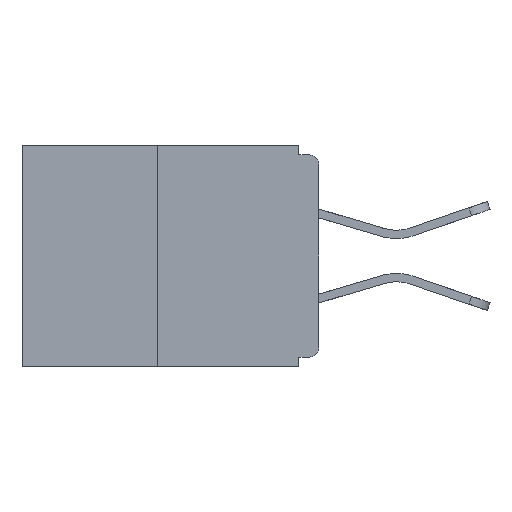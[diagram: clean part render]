
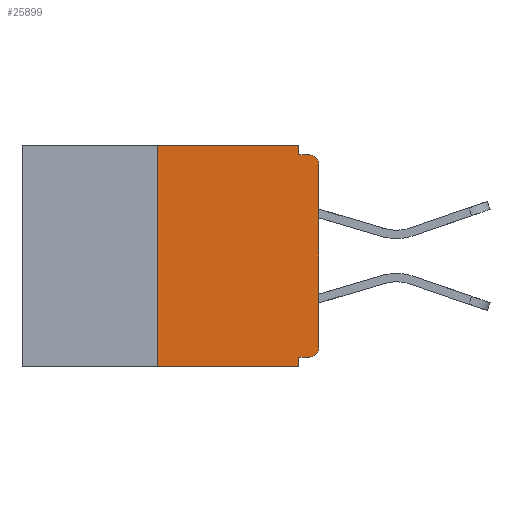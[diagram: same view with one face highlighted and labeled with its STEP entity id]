
A CAD part, left-side view. The second image highlights one B-rep face of the part: STEP entity #25899.
In plain terms, the highlighted planar face has unit normal (-1, 0, 0).
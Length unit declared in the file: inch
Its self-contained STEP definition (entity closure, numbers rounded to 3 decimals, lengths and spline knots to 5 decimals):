
#521 = EDGE_CURVE ( 'NONE', #12329, #2806, #24300, .T. ) ;
#1174 = VECTOR ( 'NONE', #25346, 39.37008 ) ;
#1480 = FACE_OUTER_BOUND ( 'NONE', #10178, .T. ) ;
#1652 = LINE ( 'NONE', #28042, #18317 ) ;
#1727 = DIRECTION ( 'NONE',  ( 0., 0., -1. ) ) ;
#1954 = DIRECTION ( 'NONE',  ( 0., -1., 0. ) ) ;
#2052 = CARTESIAN_POINT ( 'NONE',  ( 0., 0.25, 0. ) ) ;
#2169 = CARTESIAN_POINT ( 'NONE',  ( 0., 0.015, -0.313 ) ) ;
#2304 = ORIENTED_EDGE ( 'NONE', *, *, #11533, .F. ) ;
#2383 = ORIENTED_EDGE ( 'NONE', *, *, #22090, .F. ) ;
#2662 = VECTOR ( 'NONE', #10454, 39.37008 ) ;
#2806 = VERTEX_POINT ( 'NONE', #19488 ) ;
#2908 = LINE ( 'NONE', #6083, #15517 ) ;
#3956 = VERTEX_POINT ( 'NONE', #2052 ) ;
#6083 = CARTESIAN_POINT ( 'NONE',  ( 0., 0., -0.328 ) ) ;
#6183 = VECTOR ( 'NONE', #1954, 39.37008 ) ;
#6879 = ORIENTED_EDGE ( 'NONE', *, *, #10388, .T. ) ;
#7235 = VERTEX_POINT ( 'NONE', #14706 ) ;
#7419 = ORIENTED_EDGE ( 'NONE', *, *, #22670, .T. ) ;
#7583 = DIRECTION ( 'NONE',  ( -1., 0., 0. ) ) ;
#7981 = VERTEX_POINT ( 'NONE', #23427 ) ;
#8215 = EDGE_CURVE ( 'NONE', #3956, #20447, #26000, .T. ) ;
#8284 = CARTESIAN_POINT ( 'NONE',  ( 0., 0.031, 0. ) ) ;
#8979 = DIRECTION ( 'NONE',  ( 0., -1., 0. ) ) ;
#9895 = CARTESIAN_POINT ( 'NONE',  ( 0., 0., -0.313 ) ) ;
#10178 = EDGE_LOOP ( 'NONE', ( #18724, #25933, #14239, #18977, #2304, #7419, #6879, #22440, #22912, #2383 ) ) ;
#10388 = EDGE_CURVE ( 'NONE', #26975, #7235, #1652, .T. ) ;
#10442 = EDGE_CURVE ( 'NONE', #12438, #7981, #24459, .T. ) ;
#10454 = DIRECTION ( 'NONE',  ( 0., 0., -1. ) ) ;
#10725 = DIRECTION ( 'NONE',  ( 0., 0., 1. ) ) ;
#11533 = EDGE_CURVE ( 'NONE', #14965, #11704, #2908, .T. ) ;
#11553 = CIRCLE ( 'NONE', #22673, 0.015 ) ;
#11704 = VERTEX_POINT ( 'NONE', #13342 ) ;
#12066 = EDGE_CURVE ( 'NONE', #11704, #7981, #27434, .T. ) ;
#12329 = VERTEX_POINT ( 'NONE', #24838 ) ;
#12438 = VERTEX_POINT ( 'NONE', #14237 ) ;
#13263 = DIRECTION ( 'NONE',  ( 0., 0., 1. ) ) ;
#13342 = CARTESIAN_POINT ( 'NONE',  ( 0., 0.031, -0.328 ) ) ;
#13865 = CIRCLE ( 'NONE', #25889, 0.015 ) ;
#14237 = CARTESIAN_POINT ( 'NONE',  ( 0., 0.25, -0.343 ) ) ;
#14239 = ORIENTED_EDGE ( 'NONE', *, *, #10442, .T. ) ;
#14706 = CARTESIAN_POINT ( 'NONE',  ( 0., 0., -0.03 ) ) ;
#14965 = VERTEX_POINT ( 'NONE', #16021 ) ;
#15031 = DIRECTION ( 'NONE',  ( 1., 0., 0. ) ) ;
#15081 = CARTESIAN_POINT ( 'NONE',  ( 0., 0., -0.015 ) ) ;
#15517 = VECTOR ( 'NONE', #18864, 39.37008 ) ;
#15974 = CARTESIAN_POINT ( 'NONE',  ( 0., 0.46, -0.343 ) ) ;
#16021 = CARTESIAN_POINT ( 'NONE',  ( 0., 0.015, -0.328 ) ) ;
#16109 = VECTOR ( 'NONE', #13263, 39.37008 ) ;
#16915 = VECTOR ( 'NONE', #18174, 39.37008 ) ;
#16919 = CARTESIAN_POINT ( 'NONE',  ( 0., 0.46, 0. ) ) ;
#17191 = DIRECTION ( 'NONE',  ( -1., 0., 0. ) ) ;
#17285 = DIRECTION ( 'NONE',  ( 0., 0., -1. ) ) ;
#17540 = CARTESIAN_POINT ( 'NONE',  ( 0., 0.25, 0. ) ) ;
#18174 = DIRECTION ( 'NONE',  ( 0., -1., 0. ) ) ;
#18317 = VECTOR ( 'NONE', #10725, 39.37008 ) ;
#18724 = ORIENTED_EDGE ( 'NONE', *, *, #8215, .F. ) ;
#18735 = CARTESIAN_POINT ( 'NONE',  ( 0., 0.031, -0.343 ) ) ;
#18864 = DIRECTION ( 'NONE',  ( 0., 1., 0. ) ) ;
#18977 = ORIENTED_EDGE ( 'NONE', *, *, #12066, .F. ) ;
#19488 = CARTESIAN_POINT ( 'NONE',  ( 0., 0.015, -0.015 ) ) ;
#20447 = VERTEX_POINT ( 'NONE', #22862 ) ;
#20507 = EDGE_CURVE ( 'NONE', #7235, #2806, #11553, .T. ) ;
#20734 = DIRECTION ( 'NONE',  ( 0., 0., -1. ) ) ;
#21605 = CARTESIAN_POINT ( 'NONE',  ( 0., 0.46, 0. ) ) ;
#21607 = LINE ( 'NONE', #17540, #16109 ) ;
#22090 = EDGE_CURVE ( 'NONE', #20447, #12329, #22106, .T. ) ;
#22106 = LINE ( 'NONE', #8284, #2662 ) ;
#22440 = ORIENTED_EDGE ( 'NONE', *, *, #20507, .T. ) ;
#22670 = EDGE_CURVE ( 'NONE', #14965, #26975, #13865, .T. ) ;
#22673 = AXIS2_PLACEMENT_3D ( 'NONE', #24858, #7583, #20734 ) ;
#22862 = CARTESIAN_POINT ( 'NONE',  ( 0., 0.031, 0. ) ) ;
#22912 = ORIENTED_EDGE ( 'NONE', *, *, #521, .F. ) ;
#23368 = AXIS2_PLACEMENT_3D ( 'NONE', #16919, #15031, #1727 ) ;
#23427 = CARTESIAN_POINT ( 'NONE',  ( 0., 0.031, -0.343 ) ) ;
#24300 = LINE ( 'NONE', #15081, #6183 ) ;
#24459 = LINE ( 'NONE', #15974, #16915 ) ;
#24838 = CARTESIAN_POINT ( 'NONE',  ( 0., 0.031, -0.015 ) ) ;
#24858 = CARTESIAN_POINT ( 'NONE',  ( 0., 0.015, -0.03 ) ) ;
#25346 = DIRECTION ( 'NONE',  ( 0., 0., -1. ) ) ;
#25409 = EDGE_CURVE ( 'NONE', #12438, #3956, #21607, .T. ) ;
#25889 = AXIS2_PLACEMENT_3D ( 'NONE', #2169, #17191, #17285 ) ;
#25899 = ADVANCED_FACE ( 'NONE', ( #1480 ), #27931, .F. ) ;
#25933 = ORIENTED_EDGE ( 'NONE', *, *, #25409, .F. ) ;
#26000 = LINE ( 'NONE', #21605, #27368 ) ;
#26975 = VERTEX_POINT ( 'NONE', #9895 ) ;
#27368 = VECTOR ( 'NONE', #8979, 39.37008 ) ;
#27434 = LINE ( 'NONE', #18735, #1174 ) ;
#27931 = PLANE ( 'NONE',  #23368 ) ;
#28042 = CARTESIAN_POINT ( 'NONE',  ( 0., 0., 0. ) ) ;
